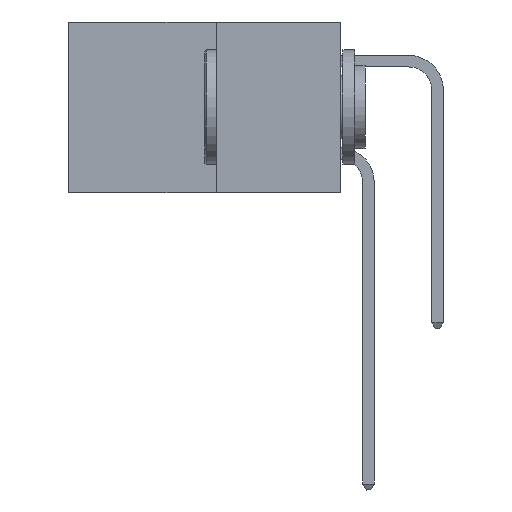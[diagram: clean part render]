
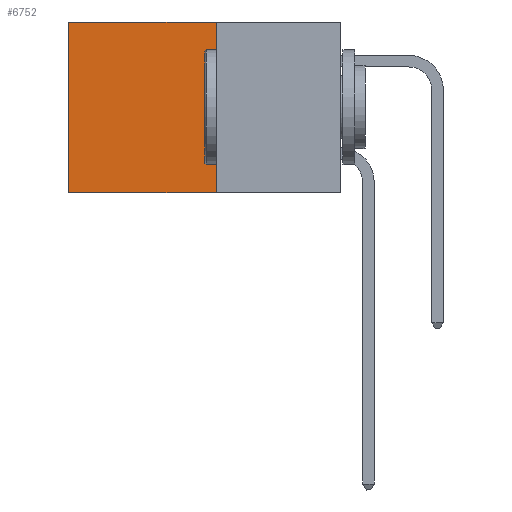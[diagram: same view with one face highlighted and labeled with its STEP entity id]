
A CAD part, left-side view. The second image highlights one B-rep face of the part: STEP entity #6752.
In plain terms, the highlighted planar face has unit normal (-1, 0, 0).
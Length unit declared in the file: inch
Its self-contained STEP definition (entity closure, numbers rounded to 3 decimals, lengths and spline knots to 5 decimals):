
#433 = CARTESIAN_POINT ( 'NONE',  ( 0.277, 0.59, 0. ) ) ;
#497 = CARTESIAN_POINT ( 'NONE',  ( 0.277, 0.59, -0.37 ) ) ;
#3848 = ORIENTED_EDGE ( 'NONE', *, *, #17933, .T. ) ;
#4950 = VECTOR ( 'NONE', #24837, 39.37008 ) ;
#5334 = DIRECTION ( 'NONE',  ( 0., 0., -1. ) ) ;
#6752 = ADVANCED_FACE ( 'NONE', ( #14692 ), #8427, .F. ) ;
#8360 = VERTEX_POINT ( 'NONE', #17647 ) ;
#8427 = PLANE ( 'NONE',  #23265 ) ;
#8995 = CARTESIAN_POINT ( 'NONE',  ( 0.277, 0.27, -0.37 ) ) ;
#10340 = CARTESIAN_POINT ( 'NONE',  ( 0.277, 0.27, -0.37 ) ) ;
#10570 = LINE ( 'NONE', #18252, #16191 ) ;
#14692 = FACE_OUTER_BOUND ( 'NONE', #25807, .T. ) ;
#15684 = DIRECTION ( 'NONE',  ( 0., 1., 0. ) ) ;
#16191 = VECTOR ( 'NONE', #18143, 39.37008 ) ;
#17647 = CARTESIAN_POINT ( 'NONE',  ( 0.277, 0.27, -0.37 ) ) ;
#17933 = EDGE_CURVE ( 'NONE', #25497, #28107, #10570, .T. ) ;
#18143 = DIRECTION ( 'NONE',  ( 0., 1., 0. ) ) ;
#18149 = CARTESIAN_POINT ( 'NONE',  ( 0.277, 0.27, -0.37 ) ) ;
#18252 = CARTESIAN_POINT ( 'NONE',  ( 0.277, 0.27, 0. ) ) ;
#18422 = LINE ( 'NONE', #497, #29562 ) ;
#18447 = VERTEX_POINT ( 'NONE', #25259 ) ;
#18829 = CARTESIAN_POINT ( 'NONE',  ( 0.277, 0.27, 0. ) ) ;
#19154 = LINE ( 'NONE', #10340, #4950 ) ;
#19874 = EDGE_CURVE ( 'NONE', #8360, #18447, #25112, .T. ) ;
#21085 = DIRECTION ( 'NONE',  ( 0., 0., -1. ) ) ;
#21187 = DIRECTION ( 'NONE',  ( 1., 0., 0. ) ) ;
#22933 = EDGE_CURVE ( 'NONE', #28107, #18447, #18422, .T. ) ;
#23265 = AXIS2_PLACEMENT_3D ( 'NONE', #8995, #21187, #21085 ) ;
#24338 = VECTOR ( 'NONE', #15684, 39.37008 ) ;
#24837 = DIRECTION ( 'NONE',  ( 0., 0., -1. ) ) ;
#25112 = LINE ( 'NONE', #18149, #24338 ) ;
#25259 = CARTESIAN_POINT ( 'NONE',  ( 0.277, 0.59, -0.37 ) ) ;
#25497 = VERTEX_POINT ( 'NONE', #18829 ) ;
#25807 = EDGE_LOOP ( 'NONE', ( #27205, #28600, #29209, #3848 ) ) ;
#27205 = ORIENTED_EDGE ( 'NONE', *, *, #22933, .T. ) ;
#28107 = VERTEX_POINT ( 'NONE', #433 ) ;
#28600 = ORIENTED_EDGE ( 'NONE', *, *, #19874, .F. ) ;
#29209 = ORIENTED_EDGE ( 'NONE', *, *, #30166, .F. ) ;
#29562 = VECTOR ( 'NONE', #5334, 39.37008 ) ;
#30166 = EDGE_CURVE ( 'NONE', #25497, #8360, #19154, .T. ) ;
